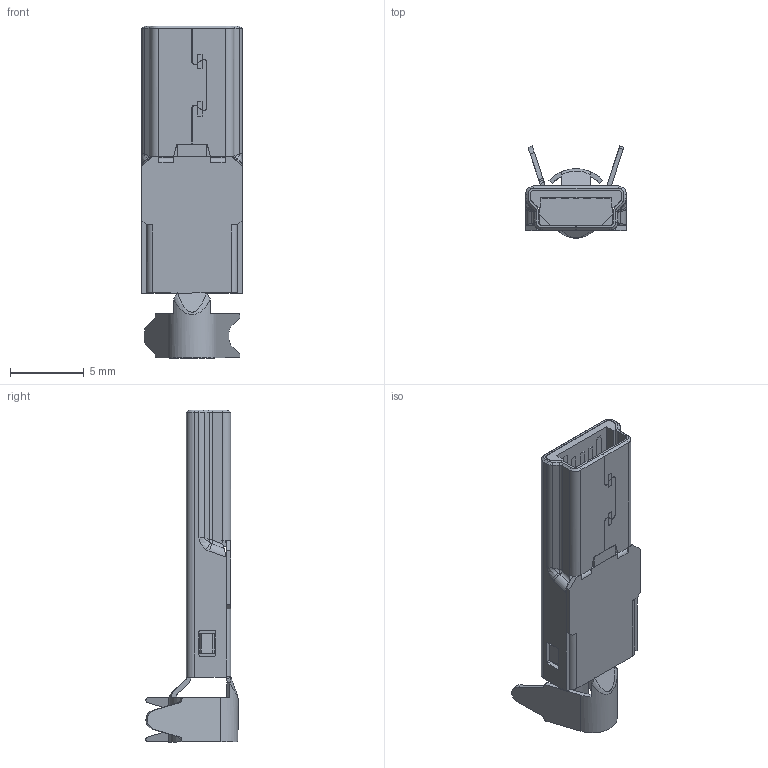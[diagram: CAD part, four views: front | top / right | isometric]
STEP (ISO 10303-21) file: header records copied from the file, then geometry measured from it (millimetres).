
FILE_DESCRIPTION (( 'STEP AP214' ), '1' );
FILE_NAME ('691G205J1A0-511 - EDAC USB Connector.STEP', '2021-01-19T16:07:36', ( '' ), ( '' ), 'SwSTEP 2.0', 'SolidWorks 2020', '' );
FILE_SCHEMA (( 'AUTOMOTIVE_DESIGN' ));
Length unit declared in the file: millimetre
Products named in the file (5): Contact 691G205JXA0-5XX; Shell1 691G205JXA0-5XX; Shell2 691G205JXA0-5XX; 691G205J1A0-511 - EDAC USB Connector; Insulator 691G205JXA0-5XX_Black
Assembly tree (4 placements, depth 2):
  691G205J1A0-511 - EDAC USB Connector
    Shell1 691G205JXA0-5XX
    Shell2 691G205JXA0-5XX
    Insulator 691G205JXA0-5XX_Black
    Contact 691G205JXA0-5XX
Bounding box: 6.8 x 6.24 x 22.5 mm (x, y, z)
Volume: 190.6 mm3; surface area: 1117.5 mm2
Topology: 8 solids, 8 shells, 439 faces, 1225 edges, 794 vertices
Faces by surface type: plane 300, cylinder 107, bspline 24, cone 8
Entity records: 15826 total; most frequent: CARTESIAN_POINT 4453, ORIENTED_EDGE 2450, DIRECTION 2154, EDGE_CURVE 1225, LINE 914, VECTOR 914, VERTEX_POINT 794, AXIS2_PLACEMENT_3D 620
